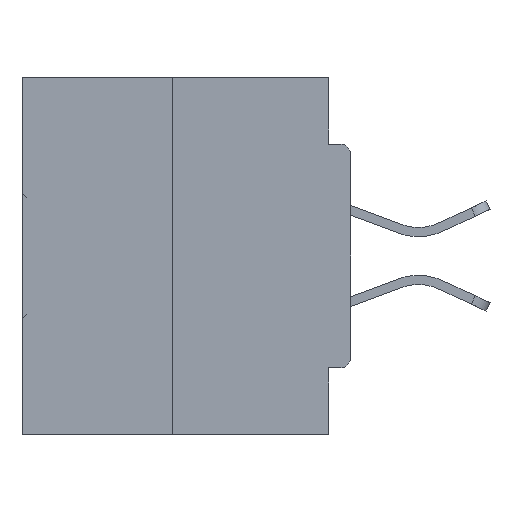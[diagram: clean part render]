
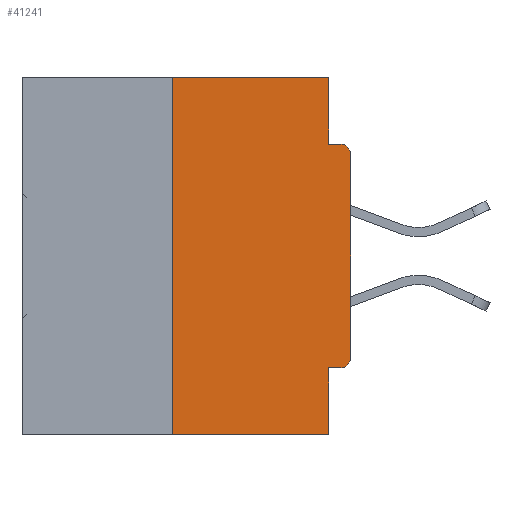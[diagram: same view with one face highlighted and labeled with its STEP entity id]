
A CAD part, left-side view. The second image highlights one B-rep face of the part: STEP entity #41241.
In plain terms, the highlighted planar face has unit normal (-1, 0, 0).
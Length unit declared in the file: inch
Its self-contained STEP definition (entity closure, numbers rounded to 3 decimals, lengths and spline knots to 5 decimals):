
#374 = CARTESIAN_POINT ( 'NONE',  ( 0., 0.46, 0. ) ) ;
#1127 = EDGE_CURVE ( 'NONE', #33636, #20082, #12684, .T. ) ;
#1673 = VERTEX_POINT ( 'NONE', #7249 ) ;
#3545 = DIRECTION ( 'NONE',  ( 0., 0., -1. ) ) ;
#3730 = ORIENTED_EDGE ( 'NONE', *, *, #13655, .T. ) ;
#4094 = ORIENTED_EDGE ( 'NONE', *, *, #1127, .F. ) ;
#4669 = ORIENTED_EDGE ( 'NONE', *, *, #34717, .F. ) ;
#4717 = CARTESIAN_POINT ( 'NONE',  ( 0., 0.46, 0. ) ) ;
#5793 = DIRECTION ( 'NONE',  ( 0., 0., -1. ) ) ;
#6649 = VECTOR ( 'NONE', #33019, 39.37008 ) ;
#6904 = ORIENTED_EDGE ( 'NONE', *, *, #40821, .T. ) ;
#7249 = CARTESIAN_POINT ( 'NONE',  ( 0., 0., -0.1085 ) ) ;
#8381 = CIRCLE ( 'NONE', #20569, 0.015 ) ;
#9600 = VECTOR ( 'NONE', #28404, 39.37008 ) ;
#9999 = EDGE_CURVE ( 'NONE', #36335, #33636, #19696, .T. ) ;
#10760 = LINE ( 'NONE', #21443, #23592 ) ;
#10920 = CARTESIAN_POINT ( 'NONE',  ( 0., 0., -0.3915 ) ) ;
#11055 = VERTEX_POINT ( 'NONE', #25414 ) ;
#11389 = DIRECTION ( 'NONE',  ( 0., 1., 0. ) ) ;
#11443 = ORIENTED_EDGE ( 'NONE', *, *, #40406, .T. ) ;
#11483 = VERTEX_POINT ( 'NONE', #21301 ) ;
#11868 = DIRECTION ( 'NONE',  ( 0., 0., -1. ) ) ;
#12199 = LINE ( 'NONE', #25856, #6649 ) ;
#12361 = EDGE_CURVE ( 'NONE', #36335, #15822, #36824, .T. ) ;
#12655 = CARTESIAN_POINT ( 'NONE',  ( 0., 0.25, 0. ) ) ;
#12684 = LINE ( 'NONE', #22945, #22678 ) ;
#13655 = EDGE_CURVE ( 'NONE', #1673, #44081, #8381, .T. ) ;
#14776 = CARTESIAN_POINT ( 'NONE',  ( 0., 0.031, -0.5 ) ) ;
#14821 = LINE ( 'NONE', #15925, #25403 ) ;
#15371 = CARTESIAN_POINT ( 'NONE',  ( 0., 0.46, -0.5 ) ) ;
#15504 = EDGE_CURVE ( 'NONE', #23749, #45361, #14821, .T. ) ;
#15820 = DIRECTION ( 'NONE',  ( -1., 0., 0. ) ) ;
#15822 = VERTEX_POINT ( 'NONE', #10920 ) ;
#15925 = CARTESIAN_POINT ( 'NONE',  ( 0., 0.25, 0. ) ) ;
#16689 = CARTESIAN_POINT ( 'NONE',  ( 0., 0.015, -0.0935 ) ) ;
#17673 = CARTESIAN_POINT ( 'NONE',  ( 0., 0.031, 0. ) ) ;
#17965 = VECTOR ( 'NONE', #11389, 39.37008 ) ;
#19328 = AXIS2_PLACEMENT_3D ( 'NONE', #29396, #29231, #43219 ) ;
#19696 = LINE ( 'NONE', #32705, #17965 ) ;
#20082 = VERTEX_POINT ( 'NONE', #14776 ) ;
#20569 = AXIS2_PLACEMENT_3D ( 'NONE', #37132, #15820, #29365 ) ;
#20669 = CARTESIAN_POINT ( 'NONE',  ( 0., 0.031, -0.4065 ) ) ;
#21273 = ORIENTED_EDGE ( 'NONE', *, *, #9999, .F. ) ;
#21301 = CARTESIAN_POINT ( 'NONE',  ( 0., 0.031, -0.0935 ) ) ;
#21443 = CARTESIAN_POINT ( 'NONE',  ( 0., 0., -0.0935 ) ) ;
#22678 = VECTOR ( 'NONE', #5793, 39.37008 ) ;
#22698 = ORIENTED_EDGE ( 'NONE', *, *, #12361, .T. ) ;
#22756 = FACE_OUTER_BOUND ( 'NONE', #33043, .T. ) ;
#22945 = CARTESIAN_POINT ( 'NONE',  ( 0., 0.031, -0.5 ) ) ;
#23592 = VECTOR ( 'NONE', #24407, 39.37008 ) ;
#23749 = VERTEX_POINT ( 'NONE', #40955 ) ;
#24407 = DIRECTION ( 'NONE',  ( 0., -1., 0. ) ) ;
#25234 = EDGE_CURVE ( 'NONE', #11483, #44081, #10760, .T. ) ;
#25403 = VECTOR ( 'NONE', #40807, 39.37008 ) ;
#25414 = CARTESIAN_POINT ( 'NONE',  ( 0., 0.031, 0. ) ) ;
#25856 = CARTESIAN_POINT ( 'NONE',  ( 0., 0., 0. ) ) ;
#26018 = PLANE ( 'NONE',  #37240 ) ;
#27390 = LINE ( 'NONE', #374, #9600 ) ;
#28404 = DIRECTION ( 'NONE',  ( 0., -1., 0. ) ) ;
#29231 = DIRECTION ( 'NONE',  ( -1., 0., 0. ) ) ;
#29365 = DIRECTION ( 'NONE',  ( 0., 0., -1. ) ) ;
#29396 = CARTESIAN_POINT ( 'NONE',  ( 0., 0.015, -0.3915 ) ) ;
#30755 = CARTESIAN_POINT ( 'NONE',  ( 0., 0.015, -0.4065 ) ) ;
#32705 = CARTESIAN_POINT ( 'NONE',  ( 0., 0., -0.4065 ) ) ;
#33019 = DIRECTION ( 'NONE',  ( 0., 0., 1. ) ) ;
#33043 = EDGE_LOOP ( 'NONE', ( #4669, #39954, #11443, #4094, #21273, #22698, #6904, #3730, #39304, #33777 ) ) ;
#33636 = VERTEX_POINT ( 'NONE', #20669 ) ;
#33777 = ORIENTED_EDGE ( 'NONE', *, *, #42731, .F. ) ;
#34717 = EDGE_CURVE ( 'NONE', #45361, #11055, #27390, .T. ) ;
#34799 = VECTOR ( 'NONE', #3545, 39.37008 ) ;
#36151 = VECTOR ( 'NONE', #40236, 39.37008 ) ;
#36335 = VERTEX_POINT ( 'NONE', #30755 ) ;
#36824 = CIRCLE ( 'NONE', #19328, 0.015 ) ;
#37132 = CARTESIAN_POINT ( 'NONE',  ( 0., 0.015, -0.1085 ) ) ;
#37240 = AXIS2_PLACEMENT_3D ( 'NONE', #4717, #43412, #11868 ) ;
#37275 = LINE ( 'NONE', #15371, #36151 ) ;
#39304 = ORIENTED_EDGE ( 'NONE', *, *, #25234, .F. ) ;
#39954 = ORIENTED_EDGE ( 'NONE', *, *, #15504, .F. ) ;
#40236 = DIRECTION ( 'NONE',  ( 0., -1., 0. ) ) ;
#40406 = EDGE_CURVE ( 'NONE', #23749, #20082, #37275, .T. ) ;
#40807 = DIRECTION ( 'NONE',  ( 0., 0., 1. ) ) ;
#40821 = EDGE_CURVE ( 'NONE', #15822, #1673, #12199, .T. ) ;
#40955 = CARTESIAN_POINT ( 'NONE',  ( 0., 0.25, -0.5 ) ) ;
#41241 = ADVANCED_FACE ( 'NONE', ( #22756 ), #26018, .F. ) ;
#42731 = EDGE_CURVE ( 'NONE', #11055, #11483, #44243, .T. ) ;
#43219 = DIRECTION ( 'NONE',  ( 0., 0., -1. ) ) ;
#43412 = DIRECTION ( 'NONE',  ( 1., 0., 0. ) ) ;
#44081 = VERTEX_POINT ( 'NONE', #16689 ) ;
#44243 = LINE ( 'NONE', #17673, #34799 ) ;
#45361 = VERTEX_POINT ( 'NONE', #12655 ) ;
